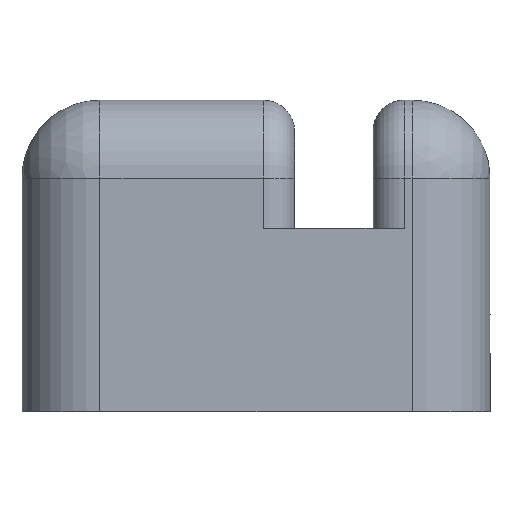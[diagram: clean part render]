
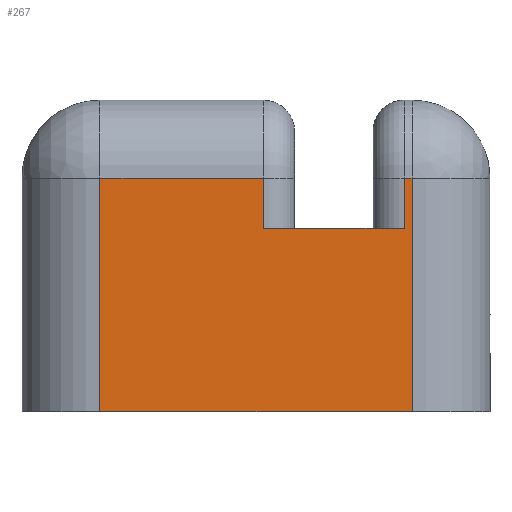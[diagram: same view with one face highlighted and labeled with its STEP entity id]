
A CAD part, left-side view. The second image highlights one B-rep face of the part: STEP entity #267.
In plain terms, the highlighted planar face has unit normal (-1, 0, 0).
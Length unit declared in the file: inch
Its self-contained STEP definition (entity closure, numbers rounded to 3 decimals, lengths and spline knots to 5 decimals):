
#267 = ADVANCED_FACE ( 'NONE', ( #6483 ), #3189, .F. ) ;
#269 = ORIENTED_EDGE ( 'NONE', *, *, #1857, .T. ) ;
#767 = EDGE_CURVE ( 'NONE', #8382, #6837, #7370, .T. ) ;
#822 = DIRECTION ( 'NONE',  ( 0., 0., 1. ) ) ;
#968 = VECTOR ( 'NONE', #3343, 39.37008 ) ;
#1065 = CARTESIAN_POINT ( 'NONE',  ( 0., 1.75, -0.25 ) ) ;
#1198 = VERTEX_POINT ( 'NONE', #5861 ) ;
#1391 = EDGE_CURVE ( 'NONE', #8382, #3890, #3088, .T. ) ;
#1540 = CARTESIAN_POINT ( 'NONE',  ( 0., 1.226, 0. ) ) ;
#1603 = DIRECTION ( 'NONE',  ( 0., -1., 0. ) ) ;
#1751 = VERTEX_POINT ( 'NONE', #4953 ) ;
#1857 = EDGE_CURVE ( 'NONE', #7854, #1198, #4227, .T. ) ;
#1873 = DIRECTION ( 'NONE',  ( 0., -1., 0. ) ) ;
#2030 = CARTESIAN_POINT ( 'NONE',  ( 0., 0.774, -0.41043 ) ) ;
#2315 = VECTOR ( 'NONE', #8381, 39.37008 ) ;
#2611 = CARTESIAN_POINT ( 'NONE',  ( 0., 0.749, 0. ) ) ;
#2881 = ORIENTED_EDGE ( 'NONE', *, *, #4481, .T. ) ;
#3010 = DIRECTION ( 'NONE',  ( 0., 0., -1. ) ) ;
#3046 = DIRECTION ( 'NONE',  ( 1., 0., 0. ) ) ;
#3088 = LINE ( 'NONE', #1540, #7666 ) ;
#3109 = ORIENTED_EDGE ( 'NONE', *, *, #4942, .T. ) ;
#3155 = EDGE_CURVE ( 'NONE', #1198, #4003, #7343, .T. ) ;
#3189 = PLANE ( 'NONE',  #6975 ) ;
#3243 = CARTESIAN_POINT ( 'NONE',  ( 0., 2., -0.25 ) ) ;
#3287 = LINE ( 'NONE', #2030, #2315 ) ;
#3343 = DIRECTION ( 'NONE',  ( 0., 1., 0. ) ) ;
#3461 = CARTESIAN_POINT ( 'NONE',  ( 0., 2., 0. ) ) ;
#3660 = EDGE_LOOP ( 'NONE', ( #9467, #2881, #9407, #3702, #3109, #6517, #269, #5464 ) ) ;
#3702 = ORIENTED_EDGE ( 'NONE', *, *, #1391, .T. ) ;
#3715 = VECTOR ( 'NONE', #1603, 39.37008 ) ;
#3890 = VERTEX_POINT ( 'NONE', #5735 ) ;
#3940 = LINE ( 'NONE', #6349, #4698 ) ;
#4003 = VERTEX_POINT ( 'NONE', #10594 ) ;
#4227 = LINE ( 'NONE', #7312, #3715 ) ;
#4411 = DIRECTION ( 'NONE',  ( 0., 0., 1. ) ) ;
#4481 = EDGE_CURVE ( 'NONE', #1751, #6837, #3287, .T. ) ;
#4689 = CARTESIAN_POINT ( 'NONE',  ( 0., 0.774, -0.41043 ) ) ;
#4698 = VECTOR ( 'NONE', #7146, 39.37008 ) ;
#4880 = CARTESIAN_POINT ( 'NONE',  ( 0., 1.226, -0.41043 ) ) ;
#4942 = EDGE_CURVE ( 'NONE', #3890, #8497, #3940, .T. ) ;
#4953 = CARTESIAN_POINT ( 'NONE',  ( 0., 0.774, -0.25 ) ) ;
#5422 = LINE ( 'NONE', #3243, #968 ) ;
#5464 = ORIENTED_EDGE ( 'NONE', *, *, #3155, .T. ) ;
#5735 = CARTESIAN_POINT ( 'NONE',  ( 0., 1.226, -0.25 ) ) ;
#5861 = CARTESIAN_POINT ( 'NONE',  ( 0., 0.749, -1. ) ) ;
#6058 = VECTOR ( 'NONE', #10623, 39.37008 ) ;
#6349 = CARTESIAN_POINT ( 'NONE',  ( 0., 2., -0.25 ) ) ;
#6483 = FACE_OUTER_BOUND ( 'NONE', #3660, .T. ) ;
#6517 = ORIENTED_EDGE ( 'NONE', *, *, #10516, .T. ) ;
#6520 = EDGE_CURVE ( 'NONE', #4003, #1751, #5422, .T. ) ;
#6837 = VERTEX_POINT ( 'NONE', #4689 ) ;
#6975 = AXIS2_PLACEMENT_3D ( 'NONE', #3461, #3046, #3010 ) ;
#7146 = DIRECTION ( 'NONE',  ( 0., 1., 0. ) ) ;
#7312 = CARTESIAN_POINT ( 'NONE',  ( 0., 2., -1. ) ) ;
#7343 = LINE ( 'NONE', #2611, #7688 ) ;
#7370 = LINE ( 'NONE', #7607, #7878 ) ;
#7607 = CARTESIAN_POINT ( 'NONE',  ( 0., 0., -0.41043 ) ) ;
#7666 = VECTOR ( 'NONE', #4411, 39.37008 ) ;
#7688 = VECTOR ( 'NONE', #822, 39.37008 ) ;
#7854 = VERTEX_POINT ( 'NONE', #10624 ) ;
#7878 = VECTOR ( 'NONE', #1873, 39.37008 ) ;
#8381 = DIRECTION ( 'NONE',  ( 0., 0., -1. ) ) ;
#8382 = VERTEX_POINT ( 'NONE', #4880 ) ;
#8497 = VERTEX_POINT ( 'NONE', #1065 ) ;
#8831 = LINE ( 'NONE', #9729, #6058 ) ;
#9407 = ORIENTED_EDGE ( 'NONE', *, *, #767, .F. ) ;
#9467 = ORIENTED_EDGE ( 'NONE', *, *, #6520, .T. ) ;
#9729 = CARTESIAN_POINT ( 'NONE',  ( 0., 1.75, 0. ) ) ;
#10516 = EDGE_CURVE ( 'NONE', #8497, #7854, #8831, .T. ) ;
#10594 = CARTESIAN_POINT ( 'NONE',  ( 0., 0.749, -0.25 ) ) ;
#10623 = DIRECTION ( 'NONE',  ( 0., 0., -1. ) ) ;
#10624 = CARTESIAN_POINT ( 'NONE',  ( 0., 1.75, -1. ) ) ;
